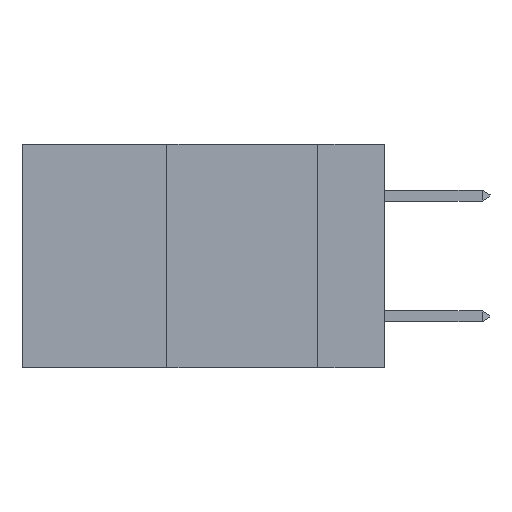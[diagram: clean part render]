
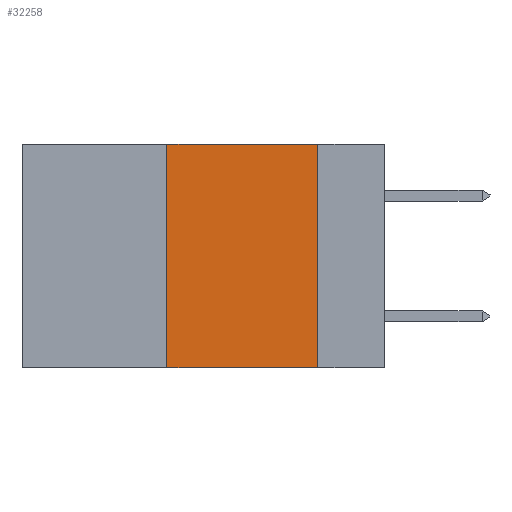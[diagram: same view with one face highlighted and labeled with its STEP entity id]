
A CAD part, left-side view. The second image highlights one B-rep face of the part: STEP entity #32258.
In plain terms, the highlighted planar face has unit normal (-1, 0, 0).
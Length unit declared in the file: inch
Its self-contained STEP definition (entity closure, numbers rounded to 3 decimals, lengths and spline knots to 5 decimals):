
#2432 = LINE ( 'NONE', #29447, #18540 ) ;
#2649 = PLANE ( 'NONE',  #11426 ) ;
#2892 = CARTESIAN_POINT ( 'NONE',  ( 0., 0.6, 0. ) ) ;
#4298 = CARTESIAN_POINT ( 'NONE',  ( 0., 0.6, -0.37 ) ) ;
#7404 = LINE ( 'NONE', #4298, #13756 ) ;
#7987 = DIRECTION ( 'NONE',  ( 1., 0., 0. ) ) ;
#8396 = EDGE_CURVE ( 'NONE', #34534, #18467, #2432, .T. ) ;
#8665 = EDGE_LOOP ( 'NONE', ( #11142, #14006, #19564, #13041 ) ) ;
#10003 = DIRECTION ( 'NONE',  ( 0., -1., 0. ) ) ;
#11142 = ORIENTED_EDGE ( 'NONE', *, *, #30819, .F. ) ;
#11295 = CARTESIAN_POINT ( 'NONE',  ( 0., 0.11, 0. ) ) ;
#11426 = AXIS2_PLACEMENT_3D ( 'NONE', #2892, #7987, #32344 ) ;
#12448 = CARTESIAN_POINT ( 'NONE',  ( 0., 0.36, 0. ) ) ;
#12861 = LINE ( 'NONE', #11295, #34043 ) ;
#13041 = ORIENTED_EDGE ( 'NONE', *, *, #30395, .T. ) ;
#13756 = VECTOR ( 'NONE', #10003, 39.37008 ) ;
#14006 = ORIENTED_EDGE ( 'NONE', *, *, #8396, .F. ) ;
#15462 = LINE ( 'NONE', #12448, #18408 ) ;
#16791 = CARTESIAN_POINT ( 'NONE',  ( 0., 0.36, -0.37 ) ) ;
#17559 = DIRECTION ( 'NONE',  ( 0., 0., 1. ) ) ;
#18408 = VECTOR ( 'NONE', #17559, 39.37008 ) ;
#18439 = CARTESIAN_POINT ( 'NONE',  ( 0., 0.36, 0. ) ) ;
#18467 = VERTEX_POINT ( 'NONE', #28046 ) ;
#18540 = VECTOR ( 'NONE', #32278, 39.37008 ) ;
#19343 = EDGE_CURVE ( 'NONE', #28920, #34534, #15462, .T. ) ;
#19564 = ORIENTED_EDGE ( 'NONE', *, *, #19343, .F. ) ;
#23369 = FACE_OUTER_BOUND ( 'NONE', #8665, .T. ) ;
#26373 = CARTESIAN_POINT ( 'NONE',  ( 0., 0.11, -0.37 ) ) ;
#28046 = CARTESIAN_POINT ( 'NONE',  ( 0., 0.11, 0. ) ) ;
#28920 = VERTEX_POINT ( 'NONE', #16791 ) ;
#29447 = CARTESIAN_POINT ( 'NONE',  ( 0., 0.6, 0. ) ) ;
#30334 = DIRECTION ( 'NONE',  ( 0., 0., -1. ) ) ;
#30395 = EDGE_CURVE ( 'NONE', #28920, #34600, #7404, .T. ) ;
#30819 = EDGE_CURVE ( 'NONE', #18467, #34600, #12861, .T. ) ;
#32258 = ADVANCED_FACE ( 'NONE', ( #23369 ), #2649, .F. ) ;
#32278 = DIRECTION ( 'NONE',  ( 0., -1., 0. ) ) ;
#32344 = DIRECTION ( 'NONE',  ( 0., 0., -1. ) ) ;
#34043 = VECTOR ( 'NONE', #30334, 39.37008 ) ;
#34534 = VERTEX_POINT ( 'NONE', #18439 ) ;
#34600 = VERTEX_POINT ( 'NONE', #26373 ) ;
